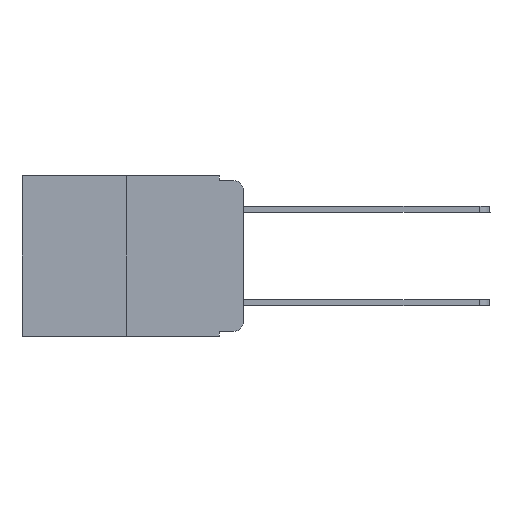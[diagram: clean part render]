
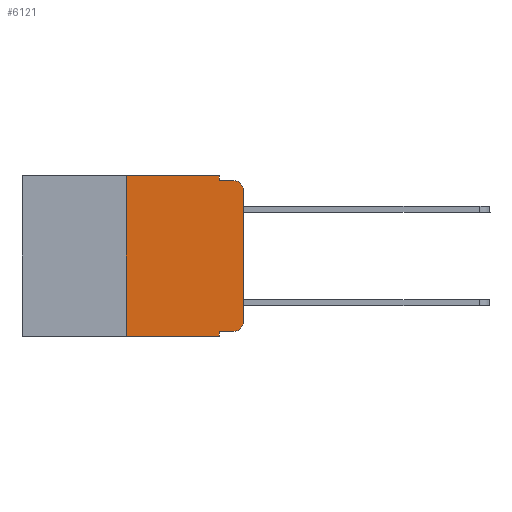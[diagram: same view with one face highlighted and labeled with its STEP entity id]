
A CAD part, left-side view. The second image highlights one B-rep face of the part: STEP entity #6121.
In plain terms, the highlighted planar face has unit normal (-1, 0, 0).
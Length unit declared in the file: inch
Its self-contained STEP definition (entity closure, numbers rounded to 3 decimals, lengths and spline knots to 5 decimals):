
#25 = CIRCLE ( 'NONE', #5205, 0.02 ) ;
#391 = DIRECTION ( 'NONE',  ( 0., -1., 0. ) ) ;
#879 = VERTEX_POINT ( 'NONE', #11325 ) ;
#972 = VECTOR ( 'NONE', #5382, 39.37008 ) ;
#1279 = DIRECTION ( 'NONE',  ( 0., 0., 1. ) ) ;
#1391 = EDGE_CURVE ( 'NONE', #3875, #12706, #10049, .T. ) ;
#1838 = VERTEX_POINT ( 'NONE', #10720 ) ;
#1964 = CARTESIAN_POINT ( 'NONE',  ( 0., 0.25, 0. ) ) ;
#2047 = VECTOR ( 'NONE', #16921, 39.37008 ) ;
#2426 = LINE ( 'NONE', #12652, #14790 ) ;
#2697 = PLANE ( 'NONE',  #6411 ) ;
#2768 = LINE ( 'NONE', #11332, #17615 ) ;
#2956 = LINE ( 'NONE', #3915, #2047 ) ;
#3433 = VECTOR ( 'NONE', #14324, 39.37008 ) ;
#3724 = EDGE_CURVE ( 'NONE', #18237, #1838, #11536, .T. ) ;
#3875 = VERTEX_POINT ( 'NONE', #1964 ) ;
#3915 = CARTESIAN_POINT ( 'NONE',  ( 0., 0.051, 0. ) ) ;
#3993 = CARTESIAN_POINT ( 'NONE',  ( 0., 0.02, -0.03 ) ) ;
#4466 = EDGE_CURVE ( 'NONE', #12706, #18237, #2956, .T. ) ;
#5205 = AXIS2_PLACEMENT_3D ( 'NONE', #3993, #16867, #11220 ) ;
#5318 = VECTOR ( 'NONE', #391, 39.37008 ) ;
#5382 = DIRECTION ( 'NONE',  ( 0., -1., 0. ) ) ;
#5715 = LINE ( 'NONE', #12398, #7083 ) ;
#6121 = ADVANCED_FACE ( 'NONE', ( #7066 ), #2697, .F. ) ;
#6278 = ORIENTED_EDGE ( 'NONE', *, *, #11463, .F. ) ;
#6347 = ORIENTED_EDGE ( 'NONE', *, *, #15314, .T. ) ;
#6411 = AXIS2_PLACEMENT_3D ( 'NONE', #7005, #9888, #14079 ) ;
#6711 = VERTEX_POINT ( 'NONE', #8178 ) ;
#7005 = CARTESIAN_POINT ( 'NONE',  ( 0., 0.473, 0. ) ) ;
#7066 = FACE_OUTER_BOUND ( 'NONE', #10953, .T. ) ;
#7083 = VECTOR ( 'NONE', #9610, 39.37008 ) ;
#7545 = ORIENTED_EDGE ( 'NONE', *, *, #17596, .T. ) ;
#8178 = CARTESIAN_POINT ( 'NONE',  ( 0., 0.051, -0.343 ) ) ;
#8455 = EDGE_CURVE ( 'NONE', #8692, #1838, #25, .T. ) ;
#8692 = VERTEX_POINT ( 'NONE', #12555 ) ;
#8949 = CARTESIAN_POINT ( 'NONE',  ( 0., 0.051, -0.333 ) ) ;
#9610 = DIRECTION ( 'NONE',  ( 0., 0., -1. ) ) ;
#9888 = DIRECTION ( 'NONE',  ( 1., 0., 0. ) ) ;
#10003 = CARTESIAN_POINT ( 'NONE',  ( 0., 0.051, -0.01 ) ) ;
#10049 = LINE ( 'NONE', #11919, #5318 ) ;
#10720 = CARTESIAN_POINT ( 'NONE',  ( 0., 0.02, -0.01 ) ) ;
#10953 = EDGE_LOOP ( 'NONE', ( #18522, #12948, #16682, #12423, #14657, #6278, #7545, #15546, #13385, #6347 ) ) ;
#11168 = CARTESIAN_POINT ( 'NONE',  ( 0., 0.051, -0.333 ) ) ;
#11220 = DIRECTION ( 'NONE',  ( 0., 0., -1. ) ) ;
#11325 = CARTESIAN_POINT ( 'NONE',  ( 0., 0.25, -0.343 ) ) ;
#11332 = CARTESIAN_POINT ( 'NONE',  ( 0., 0.473, -0.343 ) ) ;
#11393 = VERTEX_POINT ( 'NONE', #14547 ) ;
#11463 = EDGE_CURVE ( 'NONE', #879, #3875, #2426, .T. ) ;
#11536 = LINE ( 'NONE', #10003, #3433 ) ;
#11919 = CARTESIAN_POINT ( 'NONE',  ( 0., 0.473, 0. ) ) ;
#12393 = VECTOR ( 'NONE', #13205, 39.37008 ) ;
#12398 = CARTESIAN_POINT ( 'NONE',  ( 0., 0.051, 0. ) ) ;
#12423 = ORIENTED_EDGE ( 'NONE', *, *, #4466, .F. ) ;
#12555 = CARTESIAN_POINT ( 'NONE',  ( 0., 0., -0.03 ) ) ;
#12652 = CARTESIAN_POINT ( 'NONE',  ( 0., 0.25, 0. ) ) ;
#12677 = VERTEX_POINT ( 'NONE', #14338 ) ;
#12706 = VERTEX_POINT ( 'NONE', #18559 ) ;
#12761 = DIRECTION ( 'NONE',  ( 0., -1., 0. ) ) ;
#12896 = VERTEX_POINT ( 'NONE', #8949 ) ;
#12948 = ORIENTED_EDGE ( 'NONE', *, *, #8455, .T. ) ;
#13015 = DIRECTION ( 'NONE',  ( -1., 0., 0. ) ) ;
#13205 = DIRECTION ( 'NONE',  ( 0., 0., 1. ) ) ;
#13332 = LINE ( 'NONE', #11168, #972 ) ;
#13334 = CARTESIAN_POINT ( 'NONE',  ( 0., 0., 0. ) ) ;
#13385 = ORIENTED_EDGE ( 'NONE', *, *, #15078, .T. ) ;
#14079 = DIRECTION ( 'NONE',  ( 0., 0., -1. ) ) ;
#14287 = CARTESIAN_POINT ( 'NONE',  ( 0., 0.02, -0.313 ) ) ;
#14324 = DIRECTION ( 'NONE',  ( 0., -1., 0. ) ) ;
#14338 = CARTESIAN_POINT ( 'NONE',  ( 0., 0.02, -0.333 ) ) ;
#14425 = LINE ( 'NONE', #13334, #12393 ) ;
#14547 = CARTESIAN_POINT ( 'NONE',  ( 0., 0., -0.313 ) ) ;
#14657 = ORIENTED_EDGE ( 'NONE', *, *, #1391, .F. ) ;
#14790 = VECTOR ( 'NONE', #1279, 39.37008 ) ;
#14939 = EDGE_CURVE ( 'NONE', #12896, #6711, #5715, .T. ) ;
#15078 = EDGE_CURVE ( 'NONE', #12896, #12677, #13332, .T. ) ;
#15314 = EDGE_CURVE ( 'NONE', #12677, #11393, #18050, .T. ) ;
#15522 = AXIS2_PLACEMENT_3D ( 'NONE', #14287, #13015, #15908 ) ;
#15546 = ORIENTED_EDGE ( 'NONE', *, *, #14939, .F. ) ;
#15620 = CARTESIAN_POINT ( 'NONE',  ( 0., 0.051, -0.01 ) ) ;
#15908 = DIRECTION ( 'NONE',  ( 0., 0., -1. ) ) ;
#16682 = ORIENTED_EDGE ( 'NONE', *, *, #3724, .F. ) ;
#16867 = DIRECTION ( 'NONE',  ( -1., 0., 0. ) ) ;
#16921 = DIRECTION ( 'NONE',  ( 0., 0., -1. ) ) ;
#17596 = EDGE_CURVE ( 'NONE', #879, #6711, #2768, .T. ) ;
#17615 = VECTOR ( 'NONE', #12761, 39.37008 ) ;
#18050 = CIRCLE ( 'NONE', #15522, 0.02 ) ;
#18237 = VERTEX_POINT ( 'NONE', #15620 ) ;
#18478 = EDGE_CURVE ( 'NONE', #11393, #8692, #14425, .T. ) ;
#18522 = ORIENTED_EDGE ( 'NONE', *, *, #18478, .T. ) ;
#18559 = CARTESIAN_POINT ( 'NONE',  ( 0., 0.051, 0. ) ) ;
